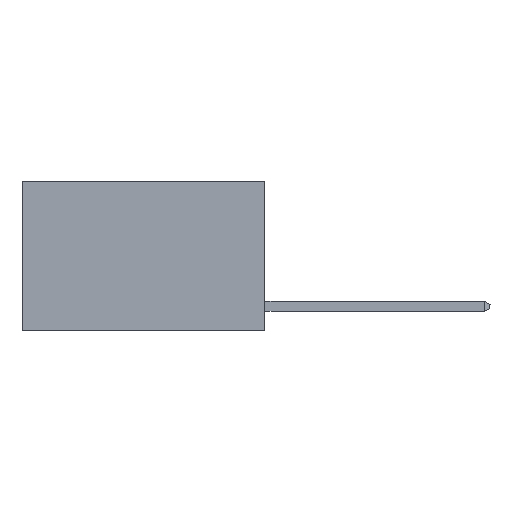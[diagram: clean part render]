
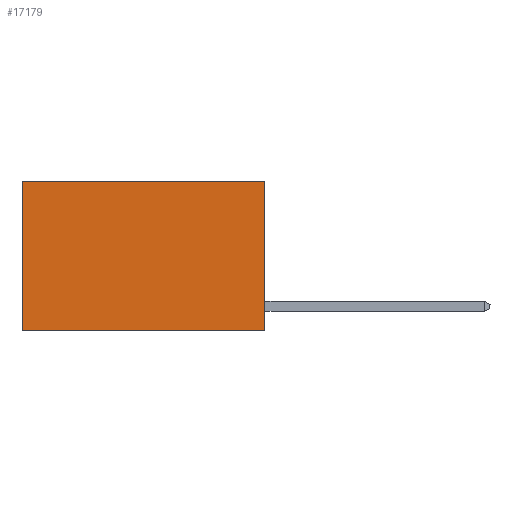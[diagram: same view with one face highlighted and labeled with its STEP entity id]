
A CAD part, left-side view. The second image highlights one B-rep face of the part: STEP entity #17179.
In plain terms, the highlighted planar face has unit normal (-1, 0, 0).
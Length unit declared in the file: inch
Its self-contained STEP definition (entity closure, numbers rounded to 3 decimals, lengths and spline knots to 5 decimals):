
#1275 = ORIENTED_EDGE ( 'NONE', *, *, #18887, .T. ) ;
#1958 = DIRECTION ( 'NONE',  ( 0., 1., 0. ) ) ;
#2980 = LINE ( 'NONE', #21513, #12153 ) ;
#3070 = VECTOR ( 'NONE', #1958, 39.37008 ) ;
#3766 = DIRECTION ( 'NONE',  ( 0., 1., 0. ) ) ;
#4269 = FACE_OUTER_BOUND ( 'NONE', #9743, .T. ) ;
#4544 = DIRECTION ( 'NONE',  ( 1., 0., 0. ) ) ;
#5064 = AXIS2_PLACEMENT_3D ( 'NONE', #15489, #4544, #17246 ) ;
#5130 = CARTESIAN_POINT ( 'NONE',  ( 0.2625, 0., 0. ) ) ;
#5590 = CARTESIAN_POINT ( 'NONE',  ( 0.2625, 0., 0. ) ) ;
#6168 = VECTOR ( 'NONE', #22251, 39.37008 ) ;
#6364 = EDGE_CURVE ( 'NONE', #8811, #7087, #2980, .T. ) ;
#7087 = VERTEX_POINT ( 'NONE', #14692 ) ;
#7349 = CARTESIAN_POINT ( 'NONE',  ( 0.2625, 0.6, -0.37 ) ) ;
#7944 = LINE ( 'NONE', #14728, #3070 ) ;
#7978 = CARTESIAN_POINT ( 'NONE',  ( 0.2625, 0.6, 0. ) ) ;
#8811 = VERTEX_POINT ( 'NONE', #5130 ) ;
#9162 = VECTOR ( 'NONE', #3766, 39.37008 ) ;
#9743 = EDGE_LOOP ( 'NONE', ( #1275, #14767, #13158, #11311 ) ) ;
#11311 = ORIENTED_EDGE ( 'NONE', *, *, #22845, .T. ) ;
#12135 = EDGE_CURVE ( 'NONE', #7087, #16886, #7944, .T. ) ;
#12153 = VECTOR ( 'NONE', #14491, 39.37008 ) ;
#13158 = ORIENTED_EDGE ( 'NONE', *, *, #6364, .F. ) ;
#14491 = DIRECTION ( 'NONE',  ( 0., 0., -1. ) ) ;
#14692 = CARTESIAN_POINT ( 'NONE',  ( 0.2625, 0., -0.37 ) ) ;
#14728 = CARTESIAN_POINT ( 'NONE',  ( 0.2625, 0., -0.37 ) ) ;
#14767 = ORIENTED_EDGE ( 'NONE', *, *, #12135, .F. ) ;
#15316 = LINE ( 'NONE', #7978, #6168 ) ;
#15489 = CARTESIAN_POINT ( 'NONE',  ( 0.2625, 0., 0. ) ) ;
#16886 = VERTEX_POINT ( 'NONE', #7349 ) ;
#17179 = ADVANCED_FACE ( 'NONE', ( #4269 ), #22493, .F. ) ;
#17246 = DIRECTION ( 'NONE',  ( 0., 0., -1. ) ) ;
#18702 = LINE ( 'NONE', #5590, #9162 ) ;
#18887 = EDGE_CURVE ( 'NONE', #21519, #16886, #15316, .T. ) ;
#21386 = CARTESIAN_POINT ( 'NONE',  ( 0.2625, 0.6, 0. ) ) ;
#21513 = CARTESIAN_POINT ( 'NONE',  ( 0.2625, 0., 0. ) ) ;
#21519 = VERTEX_POINT ( 'NONE', #21386 ) ;
#22251 = DIRECTION ( 'NONE',  ( 0., 0., -1. ) ) ;
#22493 = PLANE ( 'NONE',  #5064 ) ;
#22845 = EDGE_CURVE ( 'NONE', #8811, #21519, #18702, .T. ) ;
